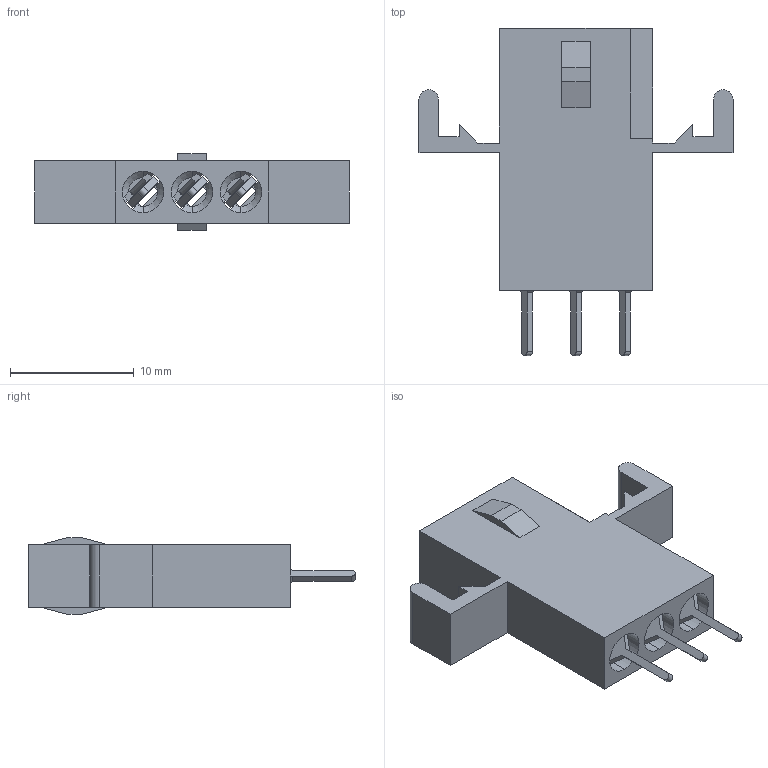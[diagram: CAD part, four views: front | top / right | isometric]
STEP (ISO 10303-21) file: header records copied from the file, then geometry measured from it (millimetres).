
FILE_DESCRIPTION (( 'STEP AP203' ), '1' );
FILE_NAME ('556-003-520-102.STEP', '2020-03-13T14:23:22', ( '' ), ( '' ), 'SwSTEP 2.0', 'SolidWorks 2016', '' );
FILE_SCHEMA (( 'CONFIG_CONTROL_DESIGN' ));
Length unit declared in the file: millimetre
Products named in the file (3): 556-210-001_556-003-000-102; 516-292-001_520 Contact; 556-003-520-102
Assembly tree (4 placements, depth 2):
  556-003-520-102
    556-210-001_556-003-000-102
    516-292-001_520 Contact  x3
Bounding box: 25.4 x 26.45 x 6.22 mm (x, y, z)
Volume: 1095.5 mm3; surface area: 2325.6 mm2
Topology: 4 solids, 4 shells, 332 faces, 954 edges, 632 vertices
Faces by surface type: plane 216, cylinder 92, bspline 18, cone 6
Entity records: 6714 total; most frequent: CARTESIAN_POINT 1482, ORIENTED_EDGE 1076, DIRECTION 950, EDGE_CURVE 538, LINE 364, VECTOR 364, VERTEX_POINT 356, AXIS2_PLACEMENT_3D 293
